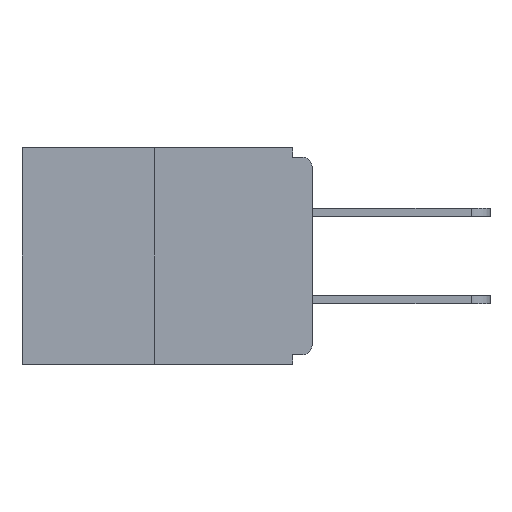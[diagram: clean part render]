
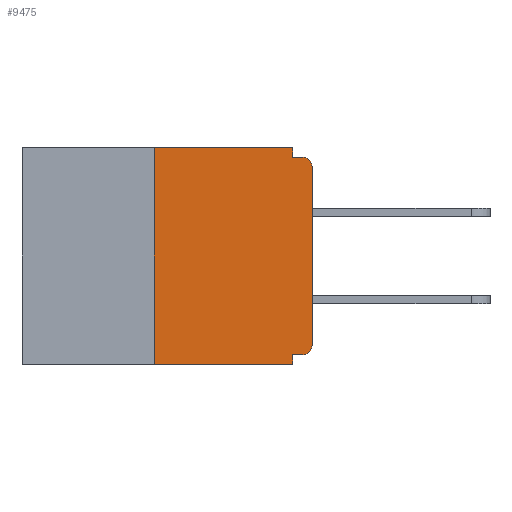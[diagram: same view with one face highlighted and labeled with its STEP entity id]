
A CAD part, left-side view. The second image highlights one B-rep face of the part: STEP entity #9475.
In plain terms, the highlighted planar face has unit normal (-1, 0, 0).
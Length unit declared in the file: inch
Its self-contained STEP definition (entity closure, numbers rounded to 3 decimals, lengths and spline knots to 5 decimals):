
#472 = CARTESIAN_POINT ( 'NONE',  ( 0., 0.46, -0.343 ) ) ;
#581 = DIRECTION ( 'NONE',  ( -1., 0., 0. ) ) ;
#1368 = EDGE_CURVE ( 'NONE', #2419, #13969, #14640, .T. ) ;
#1402 = EDGE_CURVE ( 'NONE', #8785, #13969, #2210, .T. ) ;
#1418 = CARTESIAN_POINT ( 'NONE',  ( 0., 0.25, 0. ) ) ;
#1677 = AXIS2_PLACEMENT_3D ( 'NONE', #4801, #18345, #9898 ) ;
#2210 = LINE ( 'NONE', #472, #14915 ) ;
#2419 = VERTEX_POINT ( 'NONE', #7629 ) ;
#2859 = VERTEX_POINT ( 'NONE', #21320 ) ;
#2880 = VECTOR ( 'NONE', #6437, 39.37008 ) ;
#3408 = CARTESIAN_POINT ( 'NONE',  ( 0., 0.031, -0.015 ) ) ;
#3563 = DIRECTION ( 'NONE',  ( 0., -1., 0. ) ) ;
#3848 = CARTESIAN_POINT ( 'NONE',  ( 0., 0.031, 0. ) ) ;
#3912 = CARTESIAN_POINT ( 'NONE',  ( 0., 0., -0.313 ) ) ;
#3959 = EDGE_LOOP ( 'NONE', ( #12419, #4928, #15497, #10012, #14797, #12581, #20414, #7766, #10704, #11839 ) ) ;
#4045 = DIRECTION ( 'NONE',  ( 0., 0., -1. ) ) ;
#4120 = CIRCLE ( 'NONE', #5903, 0.015 ) ;
#4494 = CARTESIAN_POINT ( 'NONE',  ( 0., 0., -0.328 ) ) ;
#4801 = CARTESIAN_POINT ( 'NONE',  ( 0., 0.46, 0. ) ) ;
#4928 = ORIENTED_EDGE ( 'NONE', *, *, #14434, .F. ) ;
#5311 = EDGE_CURVE ( 'NONE', #13193, #13893, #5763, .T. ) ;
#5319 = CIRCLE ( 'NONE', #10228, 0.015 ) ;
#5347 = LINE ( 'NONE', #7753, #13810 ) ;
#5365 = LINE ( 'NONE', #1418, #21735 ) ;
#5763 = LINE ( 'NONE', #3848, #13413 ) ;
#5816 = CARTESIAN_POINT ( 'NONE',  ( 0., 0.015, -0.313 ) ) ;
#5822 = LINE ( 'NONE', #16710, #2880 ) ;
#5903 = AXIS2_PLACEMENT_3D ( 'NONE', #21249, #12448, #21175 ) ;
#6159 = DIRECTION ( 'NONE',  ( 0., 1., 0. ) ) ;
#6437 = DIRECTION ( 'NONE',  ( 0., 0., 1. ) ) ;
#6693 = VECTOR ( 'NONE', #8779, 39.37008 ) ;
#6707 = EDGE_CURVE ( 'NONE', #14351, #2859, #4120, .T. ) ;
#7422 = LINE ( 'NONE', #4494, #10550 ) ;
#7629 = CARTESIAN_POINT ( 'NONE',  ( 0., 0.031, -0.328 ) ) ;
#7753 = CARTESIAN_POINT ( 'NONE',  ( 0., 0.46, 0. ) ) ;
#7766 = ORIENTED_EDGE ( 'NONE', *, *, #6707, .T. ) ;
#8472 = DIRECTION ( 'NONE',  ( 0., 0., 1. ) ) ;
#8712 = CARTESIAN_POINT ( 'NONE',  ( 0., 0.031, -0.343 ) ) ;
#8779 = DIRECTION ( 'NONE',  ( 0., 0., -1. ) ) ;
#8785 = VERTEX_POINT ( 'NONE', #10986 ) ;
#8789 = VERTEX_POINT ( 'NONE', #21110 ) ;
#9475 = ADVANCED_FACE ( 'NONE', ( #17399 ), #18201, .F. ) ;
#9898 = DIRECTION ( 'NONE',  ( 0., 0., -1. ) ) ;
#9942 = VERTEX_POINT ( 'NONE', #3912 ) ;
#10012 = ORIENTED_EDGE ( 'NONE', *, *, #1368, .F. ) ;
#10228 = AXIS2_PLACEMENT_3D ( 'NONE', #5816, #581, #4045 ) ;
#10424 = DIRECTION ( 'NONE',  ( 0., -1., 0. ) ) ;
#10550 = VECTOR ( 'NONE', #6159, 39.37008 ) ;
#10704 = ORIENTED_EDGE ( 'NONE', *, *, #15634, .F. ) ;
#10986 = CARTESIAN_POINT ( 'NONE',  ( 0., 0.25, -0.343 ) ) ;
#11531 = CARTESIAN_POINT ( 'NONE',  ( 0., 0.015, -0.328 ) ) ;
#11839 = ORIENTED_EDGE ( 'NONE', *, *, #5311, .F. ) ;
#11951 = DIRECTION ( 'NONE',  ( 0., 0., -1. ) ) ;
#11967 = CARTESIAN_POINT ( 'NONE',  ( 0., 0., -0.015 ) ) ;
#12262 = CARTESIAN_POINT ( 'NONE',  ( 0., 0.031, -0.343 ) ) ;
#12419 = ORIENTED_EDGE ( 'NONE', *, *, #13089, .F. ) ;
#12448 = DIRECTION ( 'NONE',  ( -1., 0., 0. ) ) ;
#12581 = ORIENTED_EDGE ( 'NONE', *, *, #15210, .T. ) ;
#13089 = EDGE_CURVE ( 'NONE', #8789, #13193, #5347, .T. ) ;
#13193 = VERTEX_POINT ( 'NONE', #15046 ) ;
#13413 = VECTOR ( 'NONE', #11951, 39.37008 ) ;
#13810 = VECTOR ( 'NONE', #18079, 39.37008 ) ;
#13893 = VERTEX_POINT ( 'NONE', #3408 ) ;
#13969 = VERTEX_POINT ( 'NONE', #12262 ) ;
#14351 = VERTEX_POINT ( 'NONE', #21356 ) ;
#14434 = EDGE_CURVE ( 'NONE', #8785, #8789, #5365, .T. ) ;
#14640 = LINE ( 'NONE', #8712, #6693 ) ;
#14797 = ORIENTED_EDGE ( 'NONE', *, *, #16044, .F. ) ;
#14915 = VECTOR ( 'NONE', #10424, 39.37008 ) ;
#15046 = CARTESIAN_POINT ( 'NONE',  ( 0., 0.031, 0. ) ) ;
#15210 = EDGE_CURVE ( 'NONE', #21429, #9942, #5319, .T. ) ;
#15497 = ORIENTED_EDGE ( 'NONE', *, *, #1402, .T. ) ;
#15634 = EDGE_CURVE ( 'NONE', #13893, #2859, #15907, .T. ) ;
#15907 = LINE ( 'NONE', #11967, #19595 ) ;
#16044 = EDGE_CURVE ( 'NONE', #21429, #2419, #7422, .T. ) ;
#16097 = EDGE_CURVE ( 'NONE', #9942, #14351, #5822, .T. ) ;
#16710 = CARTESIAN_POINT ( 'NONE',  ( 0., 0., 0. ) ) ;
#17399 = FACE_OUTER_BOUND ( 'NONE', #3959, .T. ) ;
#18079 = DIRECTION ( 'NONE',  ( 0., -1., 0. ) ) ;
#18201 = PLANE ( 'NONE',  #1677 ) ;
#18345 = DIRECTION ( 'NONE',  ( 1., 0., 0. ) ) ;
#19595 = VECTOR ( 'NONE', #3563, 39.37008 ) ;
#20414 = ORIENTED_EDGE ( 'NONE', *, *, #16097, .T. ) ;
#21110 = CARTESIAN_POINT ( 'NONE',  ( 0., 0.25, 0. ) ) ;
#21175 = DIRECTION ( 'NONE',  ( 0., 0., -1. ) ) ;
#21249 = CARTESIAN_POINT ( 'NONE',  ( 0., 0.015, -0.03 ) ) ;
#21320 = CARTESIAN_POINT ( 'NONE',  ( 0., 0.015, -0.015 ) ) ;
#21356 = CARTESIAN_POINT ( 'NONE',  ( 0., 0., -0.03 ) ) ;
#21429 = VERTEX_POINT ( 'NONE', #11531 ) ;
#21735 = VECTOR ( 'NONE', #8472, 39.37008 ) ;
